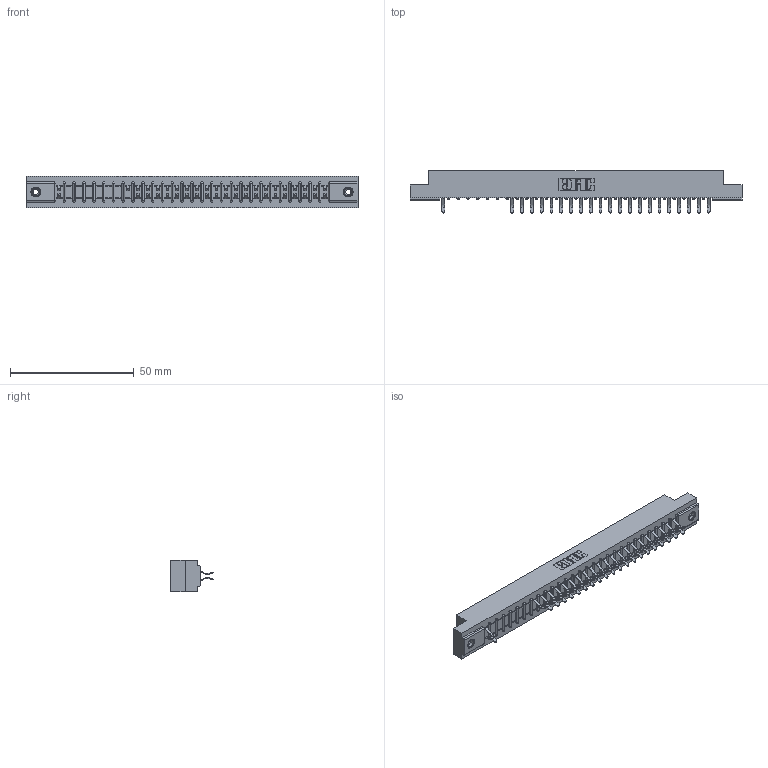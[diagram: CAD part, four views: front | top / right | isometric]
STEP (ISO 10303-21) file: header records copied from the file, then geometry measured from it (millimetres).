
FILE_DESCRIPTION (( 'STEP AP203' ), '1' );
FILE_NAME ('307-056-556-208.STEP', '2018-08-06T07:01:33', ( '' ), ( '' ), 'SwSTEP 2.0', 'SolidWorks 2016', '' );
FILE_SCHEMA (( 'CONFIG_CONTROL_DESIGN' ));
Length unit declared in the file: inch
Products named in the file (4): 307 Part_.156 Dia Mounting Holes; 307-290-001_556; 345-250-001_345-250-003-102; 307-056-556-208
Assembly tree (46 placements, depth 2):
  307-056-556-208
    307 Part_.156 Dia Mounting Holes
    307-290-001_556  x43
    345-250-001_345-250-003-102  x2
Bounding box: 133.96 x 16.97 x 12.7 mm (x, y, z)
Volume: 13963.2 mm3; surface area: 15604.2 mm2
Topology: 46 solids, 46 shells, 2487 faces, 6981 edges, 4510 vertices
Faces by surface type: plane 1599, cylinder 814, sphere 58, cone 12, torus 4
Entity records: 27499 total; most frequent: CARTESIAN_POINT 4542, ORIENTED_EDGE 4506, DIRECTION 4451, EDGE_CURVE 2253, LINE 1721, VECTOR 1721, VERTEX_POINT 1456, AXIS2_PLACEMENT_3D 1365
